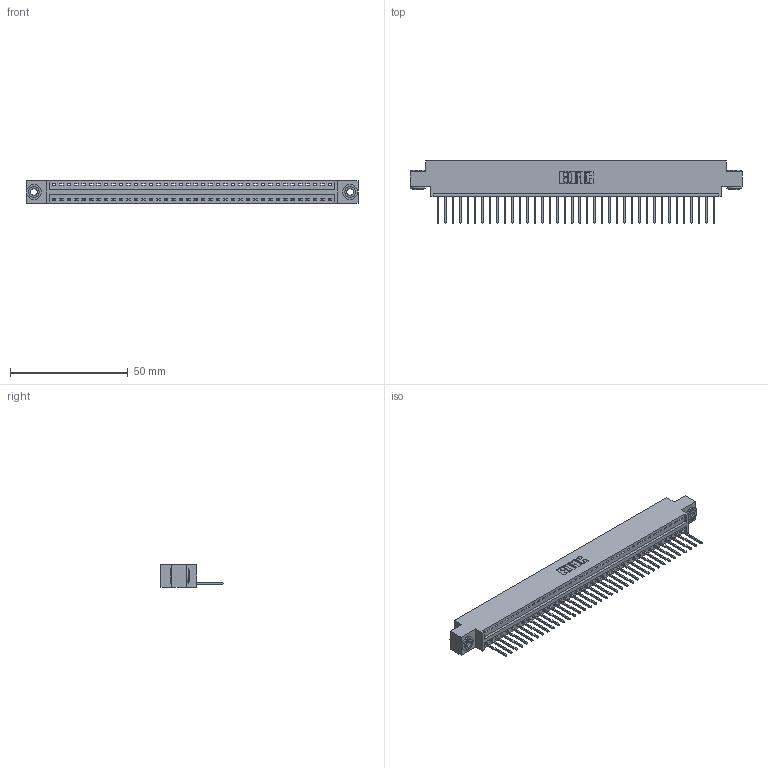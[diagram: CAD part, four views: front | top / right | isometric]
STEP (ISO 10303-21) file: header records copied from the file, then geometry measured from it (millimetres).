
FILE_DESCRIPTION (( 'STEP AP203' ), '1' );
FILE_NAME ('396-038-522-603.STEP', '2018-09-06T07:41:34', ( '' ), ( '' ), 'SwSTEP 2.0', 'SolidWorks 2016', '' );
FILE_SCHEMA (( 'CONFIG_CONTROL_DESIGN' ));
Length unit declared in the file: inch
Products named in the file (4): 346 Part_0.170 Offset - 0.156 Dia-TH; 345-292-001_345-293-122; 345-250-002_345-250-002-102; 396-038-522-603
Assembly tree (41 placements, depth 2):
  396-038-522-603
    346 Part_0.170 Offset - 0.156 Dia-TH
    345-292-001_345-293-122  x38
    345-250-002_345-250-002-102  x2
Bounding box: 141.22 x 26.42 x 9.4 mm (x, y, z)
Volume: 13360.2 mm3; surface area: 17174.8 mm2
Topology: 41 solids, 41 shells, 2368 faces, 7105 edges, 4682 vertices
Faces by surface type: plane 1610, cylinder 750, cone 8
Entity records: 24922 total; most frequent: CARTESIAN_POINT 4253, ORIENTED_EDGE 4218, DIRECTION 3787, EDGE_CURVE 2109, LINE 1801, VECTOR 1801, VERTEX_POINT 1402, AXIS2_PLACEMENT_3D 993
